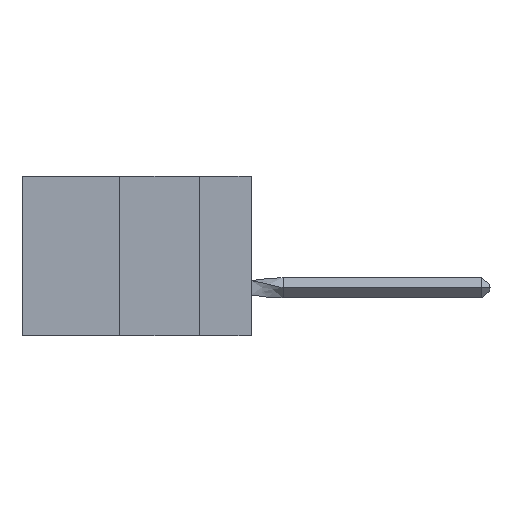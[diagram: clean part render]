
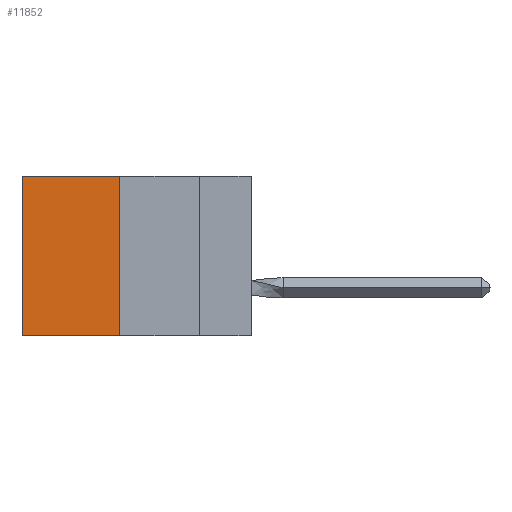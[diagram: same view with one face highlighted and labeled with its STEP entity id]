
A CAD part, left-side view. The second image highlights one B-rep face of the part: STEP entity #11852.
In plain terms, the highlighted planar face has unit normal (-1, 0, 0).
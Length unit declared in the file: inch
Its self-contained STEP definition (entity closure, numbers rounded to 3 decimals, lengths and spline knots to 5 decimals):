
#1633 = CARTESIAN_POINT ( 'NONE',  ( 0.305, 0.413, -0.5 ) ) ;
#1698 = VERTEX_POINT ( 'NONE', #3996 ) ;
#1750 = CARTESIAN_POINT ( 'NONE',  ( 0.305, 0.413, -0.5 ) ) ;
#2433 = LINE ( 'NONE', #9452, #4632 ) ;
#3844 = DIRECTION ( 'NONE',  ( 0., 1., 0. ) ) ;
#3996 = CARTESIAN_POINT ( 'NONE',  ( 0.305, 0.413, -0.5 ) ) ;
#4147 = EDGE_CURVE ( 'NONE', #21208, #20886, #2433, .T. ) ;
#4632 = VECTOR ( 'NONE', #19816, 39.37008 ) ;
#5164 = PLANE ( 'NONE',  #17488 ) ;
#5848 = EDGE_CURVE ( 'NONE', #6090, #1698, #21451, .T. ) ;
#6090 = VERTEX_POINT ( 'NONE', #7463 ) ;
#6166 = VECTOR ( 'NONE', #8310, 39.37008 ) ;
#6216 = EDGE_CURVE ( 'NONE', #6090, #21208, #18704, .T. ) ;
#6699 = VECTOR ( 'NONE', #18003, 39.37008 ) ;
#7134 = DIRECTION ( 'NONE',  ( 0., 0., -1. ) ) ;
#7463 = CARTESIAN_POINT ( 'NONE',  ( 0.305, 0.413, 0. ) ) ;
#7469 = CARTESIAN_POINT ( 'NONE',  ( 0.305, 0.72, -0.5 ) ) ;
#8310 = DIRECTION ( 'NONE',  ( 0., 0., -1. ) ) ;
#9452 = CARTESIAN_POINT ( 'NONE',  ( 0.305, 0.72, -0.5 ) ) ;
#11852 = ADVANCED_FACE ( 'NONE', ( #13195 ), #5164, .F. ) ;
#12195 = ORIENTED_EDGE ( 'NONE', *, *, #5848, .F. ) ;
#12239 = DIRECTION ( 'NONE',  ( 1., 0., 0. ) ) ;
#12923 = ORIENTED_EDGE ( 'NONE', *, *, #20220, .F. ) ;
#13195 = FACE_OUTER_BOUND ( 'NONE', #18981, .T. ) ;
#14332 = CARTESIAN_POINT ( 'NONE',  ( 0.305, 0.413, 0. ) ) ;
#15471 = CARTESIAN_POINT ( 'NONE',  ( 0.305, 0.72, 0. ) ) ;
#16609 = ORIENTED_EDGE ( 'NONE', *, *, #4147, .T. ) ;
#17167 = CARTESIAN_POINT ( 'NONE',  ( 0.305, 0.413, -0.5 ) ) ;
#17488 = AXIS2_PLACEMENT_3D ( 'NONE', #1633, #12239, #7134 ) ;
#17696 = LINE ( 'NONE', #1750, #22348 ) ;
#18003 = DIRECTION ( 'NONE',  ( 0., 1., 0. ) ) ;
#18704 = LINE ( 'NONE', #14332, #6699 ) ;
#18981 = EDGE_LOOP ( 'NONE', ( #16609, #12923, #12195, #20511 ) ) ;
#19816 = DIRECTION ( 'NONE',  ( 0., 0., -1. ) ) ;
#20220 = EDGE_CURVE ( 'NONE', #1698, #20886, #17696, .T. ) ;
#20511 = ORIENTED_EDGE ( 'NONE', *, *, #6216, .T. ) ;
#20886 = VERTEX_POINT ( 'NONE', #7469 ) ;
#21208 = VERTEX_POINT ( 'NONE', #15471 ) ;
#21451 = LINE ( 'NONE', #17167, #6166 ) ;
#22348 = VECTOR ( 'NONE', #3844, 39.37008 ) ;
